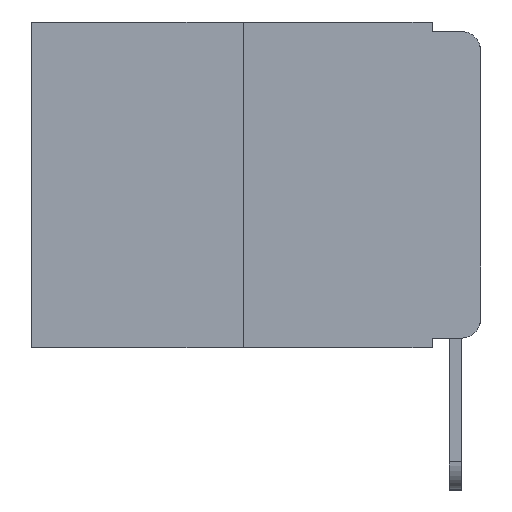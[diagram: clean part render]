
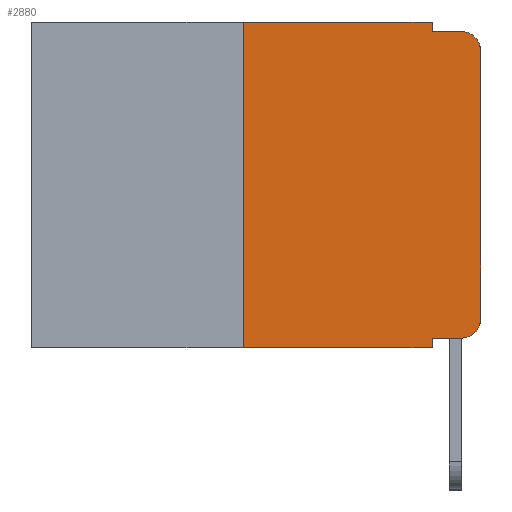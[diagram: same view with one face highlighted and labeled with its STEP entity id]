
A CAD part, left-side view. The second image highlights one B-rep face of the part: STEP entity #2880.
In plain terms, the highlighted planar face has unit normal (-1, 0, 0).
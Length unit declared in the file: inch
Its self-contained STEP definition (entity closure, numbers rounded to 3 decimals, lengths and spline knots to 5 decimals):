
#132 = DIRECTION ( 'NONE',  ( 0., -1., 0. ) ) ;
#563 = DIRECTION ( 'NONE',  ( 0., 0., 1. ) ) ;
#638 = DIRECTION ( 'NONE',  ( -1., 0., 0. ) ) ;
#673 = ORIENTED_EDGE ( 'NONE', *, *, #6456, .F. ) ;
#687 = CARTESIAN_POINT ( 'NONE',  ( 0., 0.051, -0.343 ) ) ;
#722 = AXIS2_PLACEMENT_3D ( 'NONE', #8292, #638, #9364 ) ;
#935 = VERTEX_POINT ( 'NONE', #1880 ) ;
#1317 = LINE ( 'NONE', #14390, #10263 ) ;
#1332 = VECTOR ( 'NONE', #2499, 39.37008 ) ;
#1393 = CARTESIAN_POINT ( 'NONE',  ( 0., 0.02, -0.01 ) ) ;
#1538 = CARTESIAN_POINT ( 'NONE',  ( 0., 0.473, 0. ) ) ;
#1880 = CARTESIAN_POINT ( 'NONE',  ( 0., 0.051, -0.01 ) ) ;
#1936 = ORIENTED_EDGE ( 'NONE', *, *, #6407, .T. ) ;
#1959 = DIRECTION ( 'NONE',  ( 0., 0., -1. ) ) ;
#2275 = ORIENTED_EDGE ( 'NONE', *, *, #6384, .T. ) ;
#2499 = DIRECTION ( 'NONE',  ( 0., -1., 0. ) ) ;
#2860 = VECTOR ( 'NONE', #132, 39.37008 ) ;
#2880 = ADVANCED_FACE ( 'NONE', ( #10121 ), #2890, .F. ) ;
#2890 = PLANE ( 'NONE',  #12856 ) ;
#2891 = ORIENTED_EDGE ( 'NONE', *, *, #6451, .F. ) ;
#3129 = CARTESIAN_POINT ( 'NONE',  ( 0., 0., 0. ) ) ;
#3184 = CARTESIAN_POINT ( 'NONE',  ( 0., 0.02, -0.03 ) ) ;
#3846 = ORIENTED_EDGE ( 'NONE', *, *, #6434, .F. ) ;
#3857 = ORIENTED_EDGE ( 'NONE', *, *, #6477, .T. ) ;
#3956 = CARTESIAN_POINT ( 'NONE',  ( 0., 0.02, -0.333 ) ) ;
#4056 = VECTOR ( 'NONE', #10398, 39.37008 ) ;
#4294 = VERTEX_POINT ( 'NONE', #3956 ) ;
#4424 = DIRECTION ( 'NONE',  ( 0., 0., 1. ) ) ;
#4477 = DIRECTION ( 'NONE',  ( 0., 0., -1. ) ) ;
#4591 = CARTESIAN_POINT ( 'NONE',  ( 0., 0.051, 0. ) ) ;
#4677 = VERTEX_POINT ( 'NONE', #14729 ) ;
#5666 = CIRCLE ( 'NONE', #12823, 0.02 ) ;
#5859 = CARTESIAN_POINT ( 'NONE',  ( 0., 0.051, -0.333 ) ) ;
#5981 = EDGE_CURVE ( 'NONE', #8885, #9050, #14674, .T. ) ;
#6165 = EDGE_CURVE ( 'NONE', #10306, #10174, #10932, .T. ) ;
#6384 = EDGE_CURVE ( 'NONE', #6641, #4677, #9096, .T. ) ;
#6407 = EDGE_CURVE ( 'NONE', #4677, #8803, #5666, .T. ) ;
#6414 = DIRECTION ( 'NONE',  ( 1., 0., 0. ) ) ;
#6434 = EDGE_CURVE ( 'NONE', #935, #8803, #13578, .T. ) ;
#6451 = EDGE_CURVE ( 'NONE', #9050, #935, #10589, .T. ) ;
#6453 = EDGE_CURVE ( 'NONE', #10306, #8885, #1317, .T. ) ;
#6456 = EDGE_CURVE ( 'NONE', #12158, #10174, #12940, .T. ) ;
#6475 = EDGE_CURVE ( 'NONE', #12158, #4294, #12647, .T. ) ;
#6477 = EDGE_CURVE ( 'NONE', #4294, #6641, #7342, .T. ) ;
#6535 = DIRECTION ( 'NONE',  ( 0., 0., -1. ) ) ;
#6641 = VERTEX_POINT ( 'NONE', #8708 ) ;
#7315 = CARTESIAN_POINT ( 'NONE',  ( 0., 0.25, -0.343 ) ) ;
#7342 = CIRCLE ( 'NONE', #722, 0.02 ) ;
#7716 = VECTOR ( 'NONE', #1959, 39.37008 ) ;
#7870 = CARTESIAN_POINT ( 'NONE',  ( 0., 0.25, 0. ) ) ;
#8292 = CARTESIAN_POINT ( 'NONE',  ( 0., 0.02, -0.313 ) ) ;
#8583 = CARTESIAN_POINT ( 'NONE',  ( 0., 0.473, 0. ) ) ;
#8708 = CARTESIAN_POINT ( 'NONE',  ( 0., 0., -0.313 ) ) ;
#8803 = VERTEX_POINT ( 'NONE', #1393 ) ;
#8885 = VERTEX_POINT ( 'NONE', #7870 ) ;
#9050 = VERTEX_POINT ( 'NONE', #11179 ) ;
#9096 = LINE ( 'NONE', #3129, #14207 ) ;
#9277 = CARTESIAN_POINT ( 'NONE',  ( 0., 0.051, -0.01 ) ) ;
#9317 = CARTESIAN_POINT ( 'NONE',  ( 0., 0.051, 0. ) ) ;
#9364 = DIRECTION ( 'NONE',  ( 0., 0., -1. ) ) ;
#9420 = ORIENTED_EDGE ( 'NONE', *, *, #6165, .T. ) ;
#9922 = VECTOR ( 'NONE', #12435, 39.37008 ) ;
#10121 = FACE_OUTER_BOUND ( 'NONE', #14155, .T. ) ;
#10174 = VERTEX_POINT ( 'NONE', #687 ) ;
#10263 = VECTOR ( 'NONE', #563, 39.37008 ) ;
#10306 = VERTEX_POINT ( 'NONE', #7315 ) ;
#10342 = DIRECTION ( 'NONE',  ( 0., -1., 0. ) ) ;
#10398 = DIRECTION ( 'NONE',  ( 0., 0., -1. ) ) ;
#10589 = LINE ( 'NONE', #4591, #7716 ) ;
#10781 = CARTESIAN_POINT ( 'NONE',  ( 0., 0.473, -0.343 ) ) ;
#10932 = LINE ( 'NONE', #10781, #1332 ) ;
#11179 = CARTESIAN_POINT ( 'NONE',  ( 0., 0.051, 0. ) ) ;
#11314 = DIRECTION ( 'NONE',  ( -1., 0., 0. ) ) ;
#12158 = VERTEX_POINT ( 'NONE', #12233 ) ;
#12233 = CARTESIAN_POINT ( 'NONE',  ( 0., 0.051, -0.333 ) ) ;
#12435 = DIRECTION ( 'NONE',  ( 0., -1., 0. ) ) ;
#12590 = ORIENTED_EDGE ( 'NONE', *, *, #6475, .T. ) ;
#12647 = LINE ( 'NONE', #5859, #9922 ) ;
#12823 = AXIS2_PLACEMENT_3D ( 'NONE', #3184, #11314, #4477 ) ;
#12856 = AXIS2_PLACEMENT_3D ( 'NONE', #8583, #6414, #6535 ) ;
#12915 = ORIENTED_EDGE ( 'NONE', *, *, #6453, .F. ) ;
#12940 = LINE ( 'NONE', #9317, #4056 ) ;
#13273 = VECTOR ( 'NONE', #10342, 39.37008 ) ;
#13292 = ORIENTED_EDGE ( 'NONE', *, *, #5981, .F. ) ;
#13578 = LINE ( 'NONE', #9277, #13273 ) ;
#14155 = EDGE_LOOP ( 'NONE', ( #2275, #1936, #3846, #2891, #13292, #12915, #9420, #673, #12590, #3857 ) ) ;
#14207 = VECTOR ( 'NONE', #4424, 39.37008 ) ;
#14390 = CARTESIAN_POINT ( 'NONE',  ( 0., 0.25, 0. ) ) ;
#14674 = LINE ( 'NONE', #1538, #2860 ) ;
#14729 = CARTESIAN_POINT ( 'NONE',  ( 0., 0., -0.03 ) ) ;
